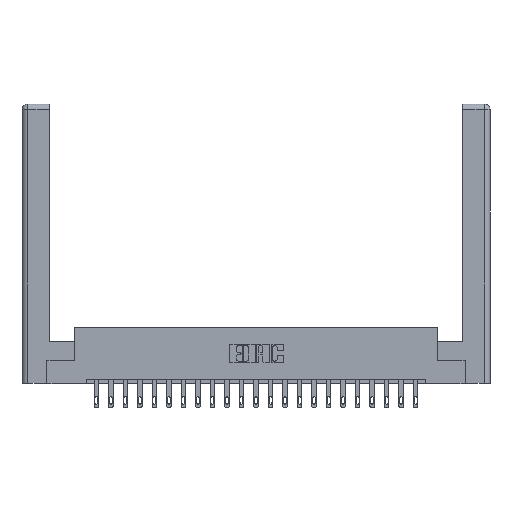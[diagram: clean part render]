
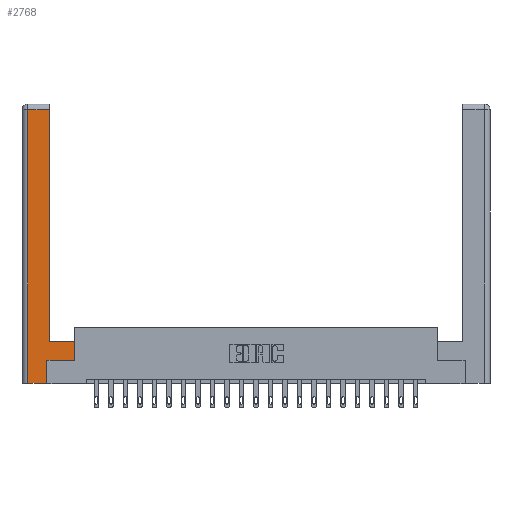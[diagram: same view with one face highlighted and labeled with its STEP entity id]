
A CAD part, top view. The second image highlights one B-rep face of the part: STEP entity #2768.
In plain terms, the highlighted planar face has unit normal (0, 0, 1).
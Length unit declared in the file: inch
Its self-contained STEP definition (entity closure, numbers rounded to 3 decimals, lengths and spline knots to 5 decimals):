
#18 = VECTOR ( 'NONE', #9912, 39.37008 ) ;
#260 = EDGE_CURVE ( 'NONE', #7297, #1858, #21352, .T. ) ;
#1235 = ORIENTED_EDGE ( 'NONE', *, *, #6638, .T. ) ;
#1469 = CARTESIAN_POINT ( 'NONE',  ( 0.565, 0.245, 0. ) ) ;
#1616 = FACE_OUTER_BOUND ( 'NONE', #12344, .T. ) ;
#1858 = VERTEX_POINT ( 'NONE', #21517 ) ;
#2330 = CARTESIAN_POINT ( 'NONE',  ( 0.0615, 0., 0. ) ) ;
#2363 = DIRECTION ( 'NONE',  ( 0., 1., 0. ) ) ;
#2768 = ADVANCED_FACE ( 'NONE', ( #1616 ), #14864, .F. ) ;
#3722 = LINE ( 'NONE', #3983, #13386 ) ;
#3983 = CARTESIAN_POINT ( 'NONE',  ( 0.265, 0., 0. ) ) ;
#4296 = CARTESIAN_POINT ( 'NONE',  ( 0., 0., 0. ) ) ;
#4524 = VERTEX_POINT ( 'NONE', #8986 ) ;
#5439 = LINE ( 'NONE', #1469, #15109 ) ;
#5450 = ORIENTED_EDGE ( 'NONE', *, *, #14141, .T. ) ;
#6228 = EDGE_CURVE ( 'NONE', #13163, #18164, #16255, .T. ) ;
#6333 = VERTEX_POINT ( 'NONE', #20786 ) ;
#6394 = DIRECTION ( 'NONE',  ( -1., 0., 0. ) ) ;
#6603 = VECTOR ( 'NONE', #9731, 39.37008 ) ;
#6638 = EDGE_CURVE ( 'NONE', #6333, #7297, #22640, .T. ) ;
#7297 = VERTEX_POINT ( 'NONE', #8605 ) ;
#7961 = CARTESIAN_POINT ( 'NONE',  ( 0.0615, 2.94, 0. ) ) ;
#7991 = EDGE_CURVE ( 'NONE', #4524, #13163, #5439, .T. ) ;
#8107 = CARTESIAN_POINT ( 'NONE',  ( 0.295, 0.45, 0. ) ) ;
#8338 = CARTESIAN_POINT ( 'NONE',  ( 0.295, 3., 0. ) ) ;
#8602 = VECTOR ( 'NONE', #22486, 39.37008 ) ;
#8605 = CARTESIAN_POINT ( 'NONE',  ( 0.0615, 2.94, 0. ) ) ;
#8986 = CARTESIAN_POINT ( 'NONE',  ( 0.265, 0.245, 0. ) ) ;
#9293 = DIRECTION ( 'NONE',  ( 1., 0., 0. ) ) ;
#9294 = ORIENTED_EDGE ( 'NONE', *, *, #13941, .T. ) ;
#9731 = DIRECTION ( 'NONE',  ( -1., 0., 0. ) ) ;
#9830 = DIRECTION ( 'NONE',  ( 0., 0., -1. ) ) ;
#9885 = AXIS2_PLACEMENT_3D ( 'NONE', #4296, #9830, #6394 ) ;
#9912 = DIRECTION ( 'NONE',  ( -1., 0., 0. ) ) ;
#9974 = VECTOR ( 'NONE', #18240, 39.37008 ) ;
#10498 = VECTOR ( 'NONE', #2363, 39.37008 ) ;
#10832 = ORIENTED_EDGE ( 'NONE', *, *, #7991, .T. ) ;
#10915 = EDGE_CURVE ( 'NONE', #1858, #20563, #3722, .T. ) ;
#11579 = LINE ( 'NONE', #16952, #18 ) ;
#12247 = CARTESIAN_POINT ( 'NONE',  ( 0.565, 0.45, 0. ) ) ;
#12344 = EDGE_LOOP ( 'NONE', ( #16415, #1235, #15991, #14633, #9294, #10832, #22767, #5450 ) ) ;
#12717 = LINE ( 'NONE', #8338, #8602 ) ;
#12872 = CARTESIAN_POINT ( 'NONE',  ( 0.265, 0.245, 0. ) ) ;
#13163 = VERTEX_POINT ( 'NONE', #14664 ) ;
#13386 = VECTOR ( 'NONE', #9293, 39.37008 ) ;
#13822 = DIRECTION ( 'NONE',  ( 1., 0., 0. ) ) ;
#13941 = EDGE_CURVE ( 'NONE', #20563, #4524, #19933, .T. ) ;
#14141 = EDGE_CURVE ( 'NONE', #18164, #17200, #11579, .T. ) ;
#14633 = ORIENTED_EDGE ( 'NONE', *, *, #10915, .T. ) ;
#14664 = CARTESIAN_POINT ( 'NONE',  ( 0.565, 0.245, 0. ) ) ;
#14864 = PLANE ( 'NONE',  #9885 ) ;
#15109 = VECTOR ( 'NONE', #13822, 39.37008 ) ;
#15801 = CARTESIAN_POINT ( 'NONE',  ( 0.265, 0., 0. ) ) ;
#15991 = ORIENTED_EDGE ( 'NONE', *, *, #260, .T. ) ;
#16255 = LINE ( 'NONE', #12247, #16803 ) ;
#16415 = ORIENTED_EDGE ( 'NONE', *, *, #19263, .T. ) ;
#16803 = VECTOR ( 'NONE', #19605, 39.37008 ) ;
#16952 = CARTESIAN_POINT ( 'NONE',  ( 0.295, 0.45, 0. ) ) ;
#17065 = CARTESIAN_POINT ( 'NONE',  ( 0.565, 0.45, 0. ) ) ;
#17200 = VERTEX_POINT ( 'NONE', #8107 ) ;
#18164 = VERTEX_POINT ( 'NONE', #17065 ) ;
#18240 = DIRECTION ( 'NONE',  ( 0., -1., 0. ) ) ;
#19263 = EDGE_CURVE ( 'NONE', #17200, #6333, #12717, .T. ) ;
#19605 = DIRECTION ( 'NONE',  ( 0., 1., 0. ) ) ;
#19933 = LINE ( 'NONE', #12872, #10498 ) ;
#20563 = VERTEX_POINT ( 'NONE', #15801 ) ;
#20786 = CARTESIAN_POINT ( 'NONE',  ( 0.295, 2.94, 0. ) ) ;
#21352 = LINE ( 'NONE', #2330, #9974 ) ;
#21517 = CARTESIAN_POINT ( 'NONE',  ( 0.0615, 0., 0. ) ) ;
#22486 = DIRECTION ( 'NONE',  ( 0., 1., 0. ) ) ;
#22640 = LINE ( 'NONE', #7961, #6603 ) ;
#22767 = ORIENTED_EDGE ( 'NONE', *, *, #6228, .T. ) ;
